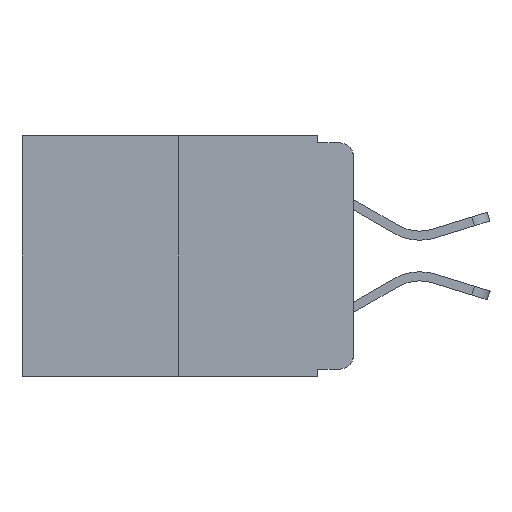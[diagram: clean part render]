
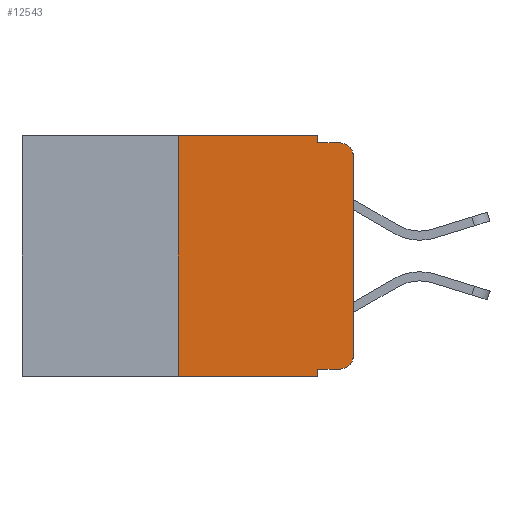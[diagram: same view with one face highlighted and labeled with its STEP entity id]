
A CAD part, left-side view. The second image highlights one B-rep face of the part: STEP entity #12543.
In plain terms, the highlighted planar face has unit normal (-1, 0, 0).
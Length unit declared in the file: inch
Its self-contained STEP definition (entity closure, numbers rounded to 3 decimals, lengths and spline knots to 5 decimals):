
#218 = LINE ( 'NONE', #9609, #13290 ) ;
#392 = ORIENTED_EDGE ( 'NONE', *, *, #16632, .F. ) ;
#745 = DIRECTION ( 'NONE',  ( 0., 0., 1. ) ) ;
#915 = CARTESIAN_POINT ( 'NONE',  ( 0., 0.02, -0.03 ) ) ;
#1052 = LINE ( 'NONE', #11789, #11310 ) ;
#1371 = CARTESIAN_POINT ( 'NONE',  ( 0., 0.473, -0.343 ) ) ;
#1418 = VECTOR ( 'NONE', #1473, 39.37008 ) ;
#1473 = DIRECTION ( 'NONE',  ( 0., -1., 0. ) ) ;
#1511 = CARTESIAN_POINT ( 'NONE',  ( 0., 0.051, 0. ) ) ;
#1541 = VERTEX_POINT ( 'NONE', #7606 ) ;
#1875 = VERTEX_POINT ( 'NONE', #7691 ) ;
#2013 = ORIENTED_EDGE ( 'NONE', *, *, #11439, .T. ) ;
#2089 = DIRECTION ( 'NONE',  ( 0., 0., -1. ) ) ;
#2092 = VERTEX_POINT ( 'NONE', #11055 ) ;
#2103 = CARTESIAN_POINT ( 'NONE',  ( 0., 0.25, 0. ) ) ;
#2241 = AXIS2_PLACEMENT_3D ( 'NONE', #8071, #10566, #15985 ) ;
#2272 = EDGE_LOOP ( 'NONE', ( #2013, #11242, #2798, #4549, #392, #6952, #13522, #7684, #2314, #6014 ) ) ;
#2277 = EDGE_CURVE ( 'NONE', #16809, #13532, #10327, .T. ) ;
#2314 = ORIENTED_EDGE ( 'NONE', *, *, #12098, .T. ) ;
#2798 = ORIENTED_EDGE ( 'NONE', *, *, #7916, .F. ) ;
#3089 = LINE ( 'NONE', #12575, #3296 ) ;
#3296 = VECTOR ( 'NONE', #4153, 39.37008 ) ;
#3946 = LINE ( 'NONE', #1371, #14350 ) ;
#3974 = AXIS2_PLACEMENT_3D ( 'NONE', #915, #17088, #9155 ) ;
#4153 = DIRECTION ( 'NONE',  ( 0., 0., -1. ) ) ;
#4437 = VERTEX_POINT ( 'NONE', #11114 ) ;
#4549 = ORIENTED_EDGE ( 'NONE', *, *, #17449, .F. ) ;
#4989 = CARTESIAN_POINT ( 'NONE',  ( 0., 0.473, 0. ) ) ;
#5236 = CARTESIAN_POINT ( 'NONE',  ( 0., 0.02, -0.01 ) ) ;
#6014 = ORIENTED_EDGE ( 'NONE', *, *, #6059, .T. ) ;
#6059 = EDGE_CURVE ( 'NONE', #8750, #4437, #12712, .T. ) ;
#6281 = CARTESIAN_POINT ( 'NONE',  ( 0., 0.051, -0.333 ) ) ;
#6617 = DIRECTION ( 'NONE',  ( 0., -1., 0. ) ) ;
#6952 = ORIENTED_EDGE ( 'NONE', *, *, #2277, .F. ) ;
#7362 = EDGE_CURVE ( 'NONE', #2092, #14475, #9053, .T. ) ;
#7606 = CARTESIAN_POINT ( 'NONE',  ( 0., 0.051, -0.01 ) ) ;
#7684 = ORIENTED_EDGE ( 'NONE', *, *, #9388, .F. ) ;
#7691 = CARTESIAN_POINT ( 'NONE',  ( 0., 0.051, -0.343 ) ) ;
#7916 = EDGE_CURVE ( 'NONE', #1541, #14475, #10787, .T. ) ;
#8071 = CARTESIAN_POINT ( 'NONE',  ( 0., 0.02, -0.313 ) ) ;
#8289 = DIRECTION ( 'NONE',  ( 0., -1., 0. ) ) ;
#8685 = DIRECTION ( 'NONE',  ( 0., 0., 1. ) ) ;
#8750 = VERTEX_POINT ( 'NONE', #9238 ) ;
#8771 = AXIS2_PLACEMENT_3D ( 'NONE', #4989, #8814, #2089 ) ;
#8814 = DIRECTION ( 'NONE',  ( 1., 0., 0. ) ) ;
#9053 = CIRCLE ( 'NONE', #3974, 0.02 ) ;
#9124 = CARTESIAN_POINT ( 'NONE',  ( 0., 0.25, 0. ) ) ;
#9155 = DIRECTION ( 'NONE',  ( 0., 0., -1. ) ) ;
#9238 = CARTESIAN_POINT ( 'NONE',  ( 0., 0.02, -0.333 ) ) ;
#9388 = EDGE_CURVE ( 'NONE', #14954, #1875, #3089, .T. ) ;
#9528 = LINE ( 'NONE', #6281, #1418 ) ;
#9558 = CARTESIAN_POINT ( 'NONE',  ( 0., 0.051, -0.333 ) ) ;
#9609 = CARTESIAN_POINT ( 'NONE',  ( 0., 0.473, 0. ) ) ;
#9645 = EDGE_CURVE ( 'NONE', #16809, #1875, #3946, .T. ) ;
#10327 = LINE ( 'NONE', #2103, #16452 ) ;
#10566 = DIRECTION ( 'NONE',  ( -1., 0., 0. ) ) ;
#10787 = LINE ( 'NONE', #13715, #14467 ) ;
#10993 = VECTOR ( 'NONE', #8685, 39.37008 ) ;
#11055 = CARTESIAN_POINT ( 'NONE',  ( 0., 0., -0.03 ) ) ;
#11114 = CARTESIAN_POINT ( 'NONE',  ( 0., 0., -0.313 ) ) ;
#11242 = ORIENTED_EDGE ( 'NONE', *, *, #7362, .T. ) ;
#11310 = VECTOR ( 'NONE', #11881, 39.37008 ) ;
#11439 = EDGE_CURVE ( 'NONE', #4437, #2092, #12521, .T. ) ;
#11789 = CARTESIAN_POINT ( 'NONE',  ( 0., 0.051, 0. ) ) ;
#11881 = DIRECTION ( 'NONE',  ( 0., 0., -1. ) ) ;
#12098 = EDGE_CURVE ( 'NONE', #14954, #8750, #9528, .T. ) ;
#12521 = LINE ( 'NONE', #16797, #10993 ) ;
#12543 = ADVANCED_FACE ( 'NONE', ( #16897 ), #17091, .F. ) ;
#12575 = CARTESIAN_POINT ( 'NONE',  ( 0., 0.051, 0. ) ) ;
#12712 = CIRCLE ( 'NONE', #2241, 0.02 ) ;
#13252 = VERTEX_POINT ( 'NONE', #1511 ) ;
#13290 = VECTOR ( 'NONE', #16555, 39.37008 ) ;
#13522 = ORIENTED_EDGE ( 'NONE', *, *, #9645, .T. ) ;
#13532 = VERTEX_POINT ( 'NONE', #9124 ) ;
#13715 = CARTESIAN_POINT ( 'NONE',  ( 0., 0.051, -0.01 ) ) ;
#14350 = VECTOR ( 'NONE', #8289, 39.37008 ) ;
#14467 = VECTOR ( 'NONE', #6617, 39.37008 ) ;
#14475 = VERTEX_POINT ( 'NONE', #5236 ) ;
#14954 = VERTEX_POINT ( 'NONE', #9558 ) ;
#15985 = DIRECTION ( 'NONE',  ( 0., 0., -1. ) ) ;
#16452 = VECTOR ( 'NONE', #745, 39.37008 ) ;
#16555 = DIRECTION ( 'NONE',  ( 0., -1., 0. ) ) ;
#16632 = EDGE_CURVE ( 'NONE', #13532, #13252, #218, .T. ) ;
#16639 = CARTESIAN_POINT ( 'NONE',  ( 0., 0.25, -0.343 ) ) ;
#16797 = CARTESIAN_POINT ( 'NONE',  ( 0., 0., 0. ) ) ;
#16809 = VERTEX_POINT ( 'NONE', #16639 ) ;
#16897 = FACE_OUTER_BOUND ( 'NONE', #2272, .T. ) ;
#17088 = DIRECTION ( 'NONE',  ( -1., 0., 0. ) ) ;
#17091 = PLANE ( 'NONE',  #8771 ) ;
#17449 = EDGE_CURVE ( 'NONE', #13252, #1541, #1052, .T. ) ;
